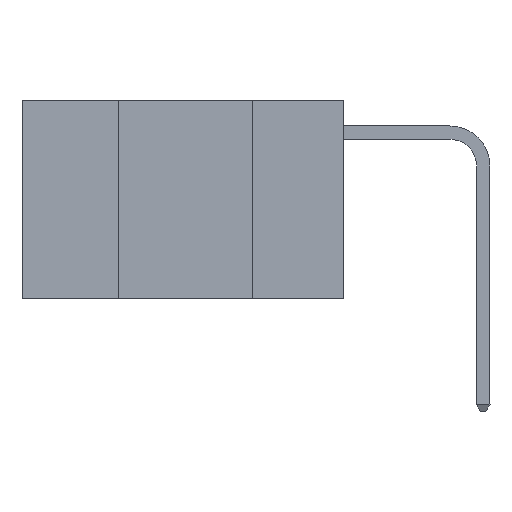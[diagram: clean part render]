
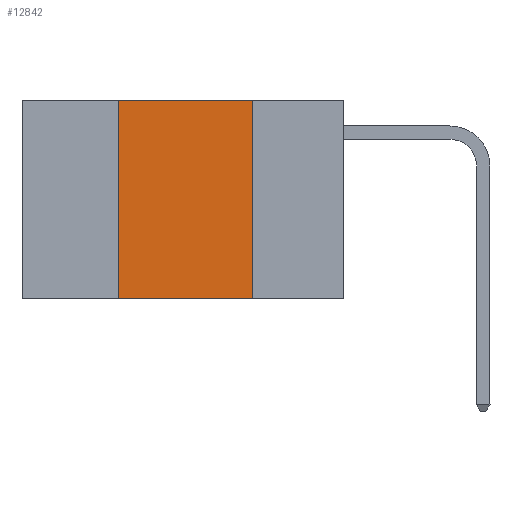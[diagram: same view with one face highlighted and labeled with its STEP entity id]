
A CAD part, left-side view. The second image highlights one B-rep face of the part: STEP entity #12842.
In plain terms, the highlighted planar face has unit normal (-1, 0, 0).
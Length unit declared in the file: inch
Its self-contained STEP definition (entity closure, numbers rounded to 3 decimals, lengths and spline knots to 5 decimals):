
#375 = VERTEX_POINT ( 'NONE', #18784 ) ;
#734 = ORIENTED_EDGE ( 'NONE', *, *, #12707, .F. ) ;
#1403 = CARTESIAN_POINT ( 'NONE',  ( 0., 0.6, 0. ) ) ;
#2626 = LINE ( 'NONE', #16393, #7132 ) ;
#3029 = VERTEX_POINT ( 'NONE', #16627 ) ;
#3494 = ORIENTED_EDGE ( 'NONE', *, *, #15667, .F. ) ;
#3849 = VERTEX_POINT ( 'NONE', #10004 ) ;
#4181 = LINE ( 'NONE', #15912, #6423 ) ;
#4304 = DIRECTION ( 'NONE',  ( 0., -1., 0. ) ) ;
#4501 = CARTESIAN_POINT ( 'NONE',  ( 0., 0.17, -0.37 ) ) ;
#6423 = VECTOR ( 'NONE', #4304, 39.37008 ) ;
#6721 = DIRECTION ( 'NONE',  ( 0., 0., -1. ) ) ;
#7132 = VECTOR ( 'NONE', #14485, 39.37008 ) ;
#7828 = LINE ( 'NONE', #9423, #20660 ) ;
#8495 = FACE_OUTER_BOUND ( 'NONE', #17830, .T. ) ;
#9423 = CARTESIAN_POINT ( 'NONE',  ( 0., 0.6, 0. ) ) ;
#9426 = ORIENTED_EDGE ( 'NONE', *, *, #19602, .F. ) ;
#10004 = CARTESIAN_POINT ( 'NONE',  ( 0., 0.17, 0. ) ) ;
#10202 = CARTESIAN_POINT ( 'NONE',  ( 0., 0.42, 0. ) ) ;
#12307 = EDGE_CURVE ( 'NONE', #3029, #22287, #4181, .T. ) ;
#12707 = EDGE_CURVE ( 'NONE', #375, #3849, #7828, .T. ) ;
#12842 = ADVANCED_FACE ( 'NONE', ( #8495 ), #13600, .F. ) ;
#13600 = PLANE ( 'NONE',  #20675 ) ;
#14485 = DIRECTION ( 'NONE',  ( 0., 0., -1. ) ) ;
#15174 = DIRECTION ( 'NONE',  ( 1., 0., 0. ) ) ;
#15667 = EDGE_CURVE ( 'NONE', #3029, #375, #19212, .T. ) ;
#15912 = CARTESIAN_POINT ( 'NONE',  ( 0., 0.6, -0.37 ) ) ;
#16057 = VECTOR ( 'NONE', #18889, 39.37008 ) ;
#16393 = CARTESIAN_POINT ( 'NONE',  ( 0., 0.17, 0. ) ) ;
#16627 = CARTESIAN_POINT ( 'NONE',  ( 0., 0.42, -0.37 ) ) ;
#17830 = EDGE_LOOP ( 'NONE', ( #9426, #734, #3494, #22296 ) ) ;
#18236 = DIRECTION ( 'NONE',  ( 0., -1., 0. ) ) ;
#18784 = CARTESIAN_POINT ( 'NONE',  ( 0., 0.42, 0. ) ) ;
#18889 = DIRECTION ( 'NONE',  ( 0., 0., 1. ) ) ;
#19212 = LINE ( 'NONE', #10202, #16057 ) ;
#19602 = EDGE_CURVE ( 'NONE', #3849, #22287, #2626, .T. ) ;
#20660 = VECTOR ( 'NONE', #18236, 39.37008 ) ;
#20675 = AXIS2_PLACEMENT_3D ( 'NONE', #1403, #15174, #6721 ) ;
#22287 = VERTEX_POINT ( 'NONE', #4501 ) ;
#22296 = ORIENTED_EDGE ( 'NONE', *, *, #12307, .T. ) ;
